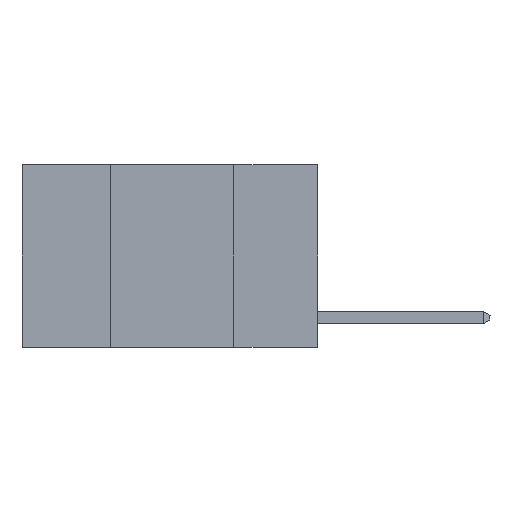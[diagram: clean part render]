
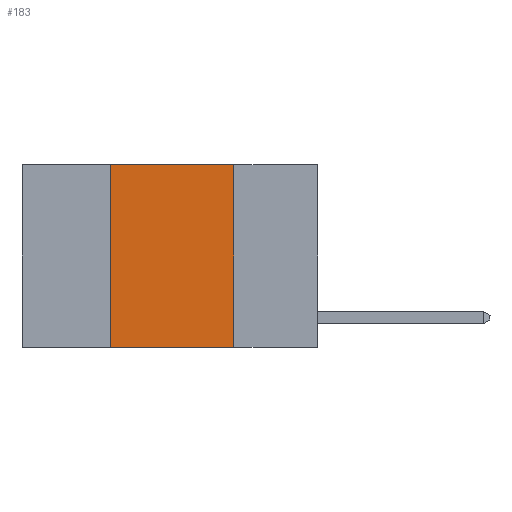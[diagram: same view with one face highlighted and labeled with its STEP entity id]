
A CAD part, left-side view. The second image highlights one B-rep face of the part: STEP entity #183.
In plain terms, the highlighted planar face has unit normal (-1, 0, 0).
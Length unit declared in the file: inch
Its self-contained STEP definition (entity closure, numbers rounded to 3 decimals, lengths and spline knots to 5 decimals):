
#183 = ADVANCED_FACE ( 'NONE', ( #9408 ), #10777, .F. ) ;
#195 = VERTEX_POINT ( 'NONE', #5761 ) ;
#1000 = VERTEX_POINT ( 'NONE', #1673 ) ;
#1296 = CARTESIAN_POINT ( 'NONE',  ( 0., 0.17, -0.37 ) ) ;
#1407 = VECTOR ( 'NONE', #5717, 39.37008 ) ;
#1522 = ORIENTED_EDGE ( 'NONE', *, *, #1967, .F. ) ;
#1673 = CARTESIAN_POINT ( 'NONE',  ( 0., 0.42, -0.37 ) ) ;
#1867 = AXIS2_PLACEMENT_3D ( 'NONE', #14548, #15821, #14605 ) ;
#1967 = EDGE_CURVE ( 'NONE', #2840, #7350, #13071, .T. ) ;
#2723 = DIRECTION ( 'NONE',  ( 0., -1., 0. ) ) ;
#2840 = VERTEX_POINT ( 'NONE', #14455 ) ;
#3192 = LINE ( 'NONE', #4885, #11894 ) ;
#3391 = ORIENTED_EDGE ( 'NONE', *, *, #7868, .T. ) ;
#3640 = EDGE_CURVE ( 'NONE', #1000, #195, #12050, .T. ) ;
#4514 = EDGE_LOOP ( 'NONE', ( #1522, #5601, #7422, #3391 ) ) ;
#4885 = CARTESIAN_POINT ( 'NONE',  ( 0., 0.6, -0.37 ) ) ;
#5175 = CARTESIAN_POINT ( 'NONE',  ( 0., 0.6, 0. ) ) ;
#5520 = CARTESIAN_POINT ( 'NONE',  ( 0., 0.17, 0. ) ) ;
#5601 = ORIENTED_EDGE ( 'NONE', *, *, #7546, .F. ) ;
#5717 = DIRECTION ( 'NONE',  ( 0., 0., 1. ) ) ;
#5761 = CARTESIAN_POINT ( 'NONE',  ( 0., 0.42, 0. ) ) ;
#6316 = DIRECTION ( 'NONE',  ( 0., -1., 0. ) ) ;
#7350 = VERTEX_POINT ( 'NONE', #1296 ) ;
#7422 = ORIENTED_EDGE ( 'NONE', *, *, #3640, .F. ) ;
#7546 = EDGE_CURVE ( 'NONE', #195, #2840, #13649, .T. ) ;
#7868 = EDGE_CURVE ( 'NONE', #1000, #7350, #3192, .T. ) ;
#8044 = VECTOR ( 'NONE', #2723, 39.37008 ) ;
#8063 = DIRECTION ( 'NONE',  ( 0., 0., -1. ) ) ;
#9408 = FACE_OUTER_BOUND ( 'NONE', #4514, .T. ) ;
#9766 = VECTOR ( 'NONE', #8063, 39.37008 ) ;
#10777 = PLANE ( 'NONE',  #1867 ) ;
#11894 = VECTOR ( 'NONE', #6316, 39.37008 ) ;
#12050 = LINE ( 'NONE', #13128, #1407 ) ;
#13071 = LINE ( 'NONE', #5520, #9766 ) ;
#13128 = CARTESIAN_POINT ( 'NONE',  ( 0., 0.42, 0. ) ) ;
#13649 = LINE ( 'NONE', #5175, #8044 ) ;
#14455 = CARTESIAN_POINT ( 'NONE',  ( 0., 0.17, 0. ) ) ;
#14548 = CARTESIAN_POINT ( 'NONE',  ( 0., 0.6, 0. ) ) ;
#14605 = DIRECTION ( 'NONE',  ( 0., 0., -1. ) ) ;
#15821 = DIRECTION ( 'NONE',  ( 1., 0., 0. ) ) ;
